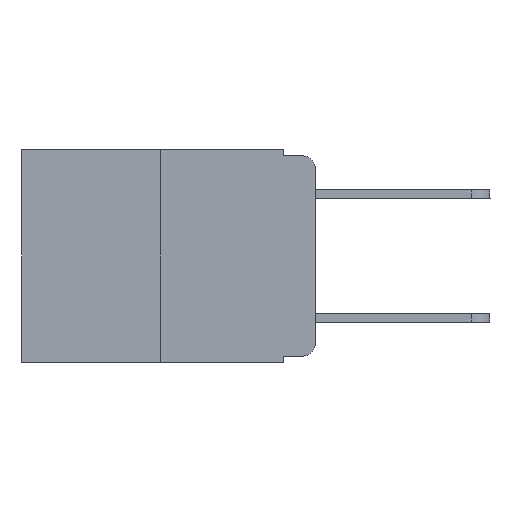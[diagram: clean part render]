
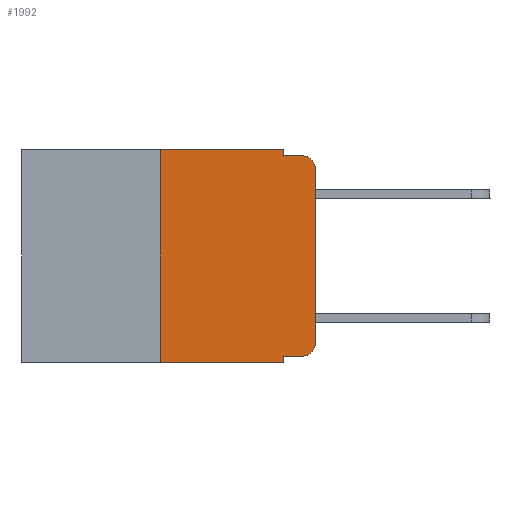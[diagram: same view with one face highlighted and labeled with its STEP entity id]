
A CAD part, left-side view. The second image highlights one B-rep face of the part: STEP entity #1992.
In plain terms, the highlighted planar face has unit normal (-1, 0, 0).
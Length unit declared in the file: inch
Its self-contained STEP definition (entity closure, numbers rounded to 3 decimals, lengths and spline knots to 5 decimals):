
#120 = LINE ( 'NONE', #828, #23200 ) ;
#259 = VERTEX_POINT ( 'NONE', #11093 ) ;
#520 = ORIENTED_EDGE ( 'NONE', *, *, #24183, .T. ) ;
#828 = CARTESIAN_POINT ( 'NONE',  ( 0., 0.051, -0.333 ) ) ;
#1251 = DIRECTION ( 'NONE',  ( -1., 0., 0. ) ) ;
#1634 = LINE ( 'NONE', #9164, #4181 ) ;
#1779 = CIRCLE ( 'NONE', #15789, 0.02 ) ;
#1813 = CARTESIAN_POINT ( 'NONE',  ( 0., 0.473, -0.343 ) ) ;
#1992 = ADVANCED_FACE ( 'NONE', ( #10824 ), #18459, .F. ) ;
#2295 = ORIENTED_EDGE ( 'NONE', *, *, #5172, .T. ) ;
#3309 = CARTESIAN_POINT ( 'NONE',  ( 0., 0.473, 0. ) ) ;
#3491 = LINE ( 'NONE', #16879, #19380 ) ;
#3596 = VERTEX_POINT ( 'NONE', #6031 ) ;
#4181 = VECTOR ( 'NONE', #5420, 39.37008 ) ;
#4198 = EDGE_CURVE ( 'NONE', #5591, #4210, #9079, .T. ) ;
#4210 = VERTEX_POINT ( 'NONE', #16704 ) ;
#4338 = DIRECTION ( 'NONE',  ( 0., 0., -1. ) ) ;
#4481 = CARTESIAN_POINT ( 'NONE',  ( 0., 0.051, -0.333 ) ) ;
#4759 = CARTESIAN_POINT ( 'NONE',  ( 0., 0.02, -0.313 ) ) ;
#4862 = EDGE_CURVE ( 'NONE', #20445, #23155, #1634, .T. ) ;
#5172 = EDGE_CURVE ( 'NONE', #20275, #3596, #1779, .T. ) ;
#5205 = EDGE_CURVE ( 'NONE', #23155, #7104, #3491, .T. ) ;
#5347 = ORIENTED_EDGE ( 'NONE', *, *, #13333, .T. ) ;
#5420 = DIRECTION ( 'NONE',  ( 0., 0., 1. ) ) ;
#5455 = AXIS2_PLACEMENT_3D ( 'NONE', #3309, #13063, #24105 ) ;
#5498 = ORIENTED_EDGE ( 'NONE', *, *, #9155, .F. ) ;
#5591 = VERTEX_POINT ( 'NONE', #4481 ) ;
#5963 = LINE ( 'NONE', #1813, #15274 ) ;
#6031 = CARTESIAN_POINT ( 'NONE',  ( 0., 0., -0.313 ) ) ;
#6052 = VERTEX_POINT ( 'NONE', #6474 ) ;
#6155 = ORIENTED_EDGE ( 'NONE', *, *, #16034, .T. ) ;
#6474 = CARTESIAN_POINT ( 'NONE',  ( 0., 0., -0.03 ) ) ;
#6969 = CARTESIAN_POINT ( 'NONE',  ( 0., 0., 0. ) ) ;
#7104 = VERTEX_POINT ( 'NONE', #9947 ) ;
#7576 = DIRECTION ( 'NONE',  ( 0., -1., 0. ) ) ;
#8588 = CARTESIAN_POINT ( 'NONE',  ( 0., 0.02, -0.03 ) ) ;
#8811 = VECTOR ( 'NONE', #8912, 39.37008 ) ;
#8912 = DIRECTION ( 'NONE',  ( 0., 0., -1. ) ) ;
#9079 = LINE ( 'NONE', #19621, #10511 ) ;
#9117 = CARTESIAN_POINT ( 'NONE',  ( 0., 0.051, -0.01 ) ) ;
#9155 = EDGE_CURVE ( 'NONE', #7104, #259, #19817, .T. ) ;
#9164 = CARTESIAN_POINT ( 'NONE',  ( 0., 0.25, 0. ) ) ;
#9416 = CIRCLE ( 'NONE', #19806, 0.02 ) ;
#9947 = CARTESIAN_POINT ( 'NONE',  ( 0., 0.051, 0. ) ) ;
#9948 = EDGE_LOOP ( 'NONE', ( #6155, #16868, #20332, #5498, #17170, #14358, #520, #20173, #5347, #2295 ) ) ;
#10423 = CARTESIAN_POINT ( 'NONE',  ( 0., 0.02, -0.01 ) ) ;
#10511 = VECTOR ( 'NONE', #19756, 39.37008 ) ;
#10762 = DIRECTION ( 'NONE',  ( 0., 0., -1. ) ) ;
#10824 = FACE_OUTER_BOUND ( 'NONE', #9948, .T. ) ;
#11093 = CARTESIAN_POINT ( 'NONE',  ( 0., 0.051, -0.01 ) ) ;
#11156 = CARTESIAN_POINT ( 'NONE',  ( 0., 0.02, -0.333 ) ) ;
#12577 = VERTEX_POINT ( 'NONE', #10423 ) ;
#12739 = DIRECTION ( 'NONE',  ( 0., -1., 0. ) ) ;
#13063 = DIRECTION ( 'NONE',  ( 1., 0., 0. ) ) ;
#13333 = EDGE_CURVE ( 'NONE', #5591, #20275, #120, .T. ) ;
#14344 = DIRECTION ( 'NONE',  ( 0., -1., 0. ) ) ;
#14358 = ORIENTED_EDGE ( 'NONE', *, *, #4862, .F. ) ;
#14540 = CARTESIAN_POINT ( 'NONE',  ( 0., 0.051, 0. ) ) ;
#14629 = LINE ( 'NONE', #9117, #15601 ) ;
#14825 = DIRECTION ( 'NONE',  ( 0., 0., 1. ) ) ;
#15274 = VECTOR ( 'NONE', #7576, 39.37008 ) ;
#15601 = VECTOR ( 'NONE', #12739, 39.37008 ) ;
#15789 = AXIS2_PLACEMENT_3D ( 'NONE', #4759, #1251, #10762 ) ;
#16034 = EDGE_CURVE ( 'NONE', #3596, #6052, #16462, .T. ) ;
#16462 = LINE ( 'NONE', #6969, #18048 ) ;
#16704 = CARTESIAN_POINT ( 'NONE',  ( 0., 0.051, -0.343 ) ) ;
#16868 = ORIENTED_EDGE ( 'NONE', *, *, #21466, .T. ) ;
#16879 = CARTESIAN_POINT ( 'NONE',  ( 0., 0.473, 0. ) ) ;
#17170 = ORIENTED_EDGE ( 'NONE', *, *, #5205, .F. ) ;
#18048 = VECTOR ( 'NONE', #14825, 39.37008 ) ;
#18459 = PLANE ( 'NONE',  #5455 ) ;
#19380 = VECTOR ( 'NONE', #20773, 39.37008 ) ;
#19621 = CARTESIAN_POINT ( 'NONE',  ( 0., 0.051, 0. ) ) ;
#19756 = DIRECTION ( 'NONE',  ( 0., 0., -1. ) ) ;
#19806 = AXIS2_PLACEMENT_3D ( 'NONE', #8588, #21490, #4338 ) ;
#19817 = LINE ( 'NONE', #14540, #8811 ) ;
#19951 = CARTESIAN_POINT ( 'NONE',  ( 0., 0.25, 0. ) ) ;
#20173 = ORIENTED_EDGE ( 'NONE', *, *, #4198, .F. ) ;
#20275 = VERTEX_POINT ( 'NONE', #11156 ) ;
#20332 = ORIENTED_EDGE ( 'NONE', *, *, #22364, .F. ) ;
#20445 = VERTEX_POINT ( 'NONE', #21053 ) ;
#20773 = DIRECTION ( 'NONE',  ( 0., -1., 0. ) ) ;
#21053 = CARTESIAN_POINT ( 'NONE',  ( 0., 0.25, -0.343 ) ) ;
#21466 = EDGE_CURVE ( 'NONE', #6052, #12577, #9416, .T. ) ;
#21490 = DIRECTION ( 'NONE',  ( -1., 0., 0. ) ) ;
#22364 = EDGE_CURVE ( 'NONE', #259, #12577, #14629, .T. ) ;
#23155 = VERTEX_POINT ( 'NONE', #19951 ) ;
#23200 = VECTOR ( 'NONE', #14344, 39.37008 ) ;
#24105 = DIRECTION ( 'NONE',  ( 0., 0., -1. ) ) ;
#24183 = EDGE_CURVE ( 'NONE', #20445, #4210, #5963, .T. ) ;
